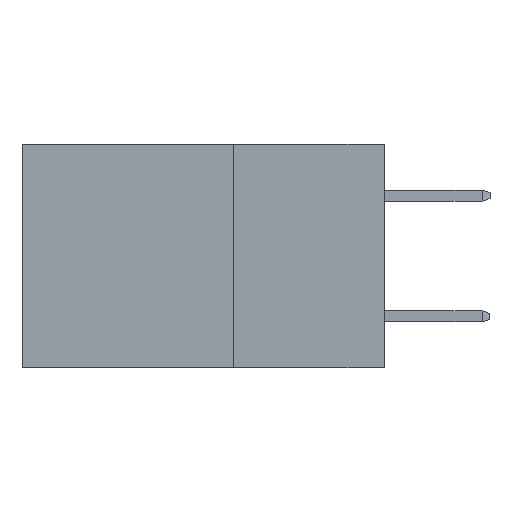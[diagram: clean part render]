
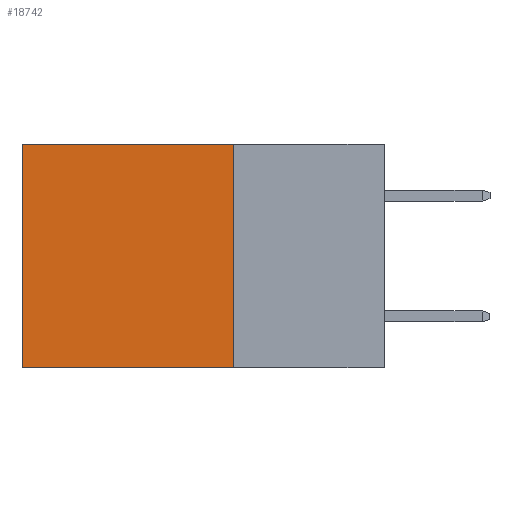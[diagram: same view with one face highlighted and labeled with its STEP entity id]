
A CAD part, left-side view. The second image highlights one B-rep face of the part: STEP entity #18742.
In plain terms, the highlighted planar face has unit normal (-1, 0, 0).
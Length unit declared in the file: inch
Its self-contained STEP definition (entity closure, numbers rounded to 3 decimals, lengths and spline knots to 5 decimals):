
#263 = PLANE ( 'NONE',  #11855 ) ;
#1219 = ORIENTED_EDGE ( 'NONE', *, *, #14883, .T. ) ;
#1270 = EDGE_CURVE ( 'NONE', #6157, #12100, #19484, .T. ) ;
#1410 = DIRECTION ( 'NONE',  ( 0., 1., 0. ) ) ;
#1471 = CARTESIAN_POINT ( 'NONE',  ( 0.298, 0.6, 0. ) ) ;
#1867 = DIRECTION ( 'NONE',  ( 1., 0., 0. ) ) ;
#2210 = VERTEX_POINT ( 'NONE', #16109 ) ;
#2574 = CARTESIAN_POINT ( 'NONE',  ( 0.298, 0.25, -0.37 ) ) ;
#3361 = VECTOR ( 'NONE', #16623, 39.37008 ) ;
#5173 = CARTESIAN_POINT ( 'NONE',  ( 0.298, 0.25, 0. ) ) ;
#6157 = VERTEX_POINT ( 'NONE', #2574 ) ;
#7993 = LINE ( 'NONE', #18135, #11607 ) ;
#8457 = CARTESIAN_POINT ( 'NONE',  ( 0.298, 0.25, -0.37 ) ) ;
#8536 = EDGE_CURVE ( 'NONE', #17518, #2210, #7993, .T. ) ;
#8876 = ORIENTED_EDGE ( 'NONE', *, *, #1270, .F. ) ;
#9138 = VECTOR ( 'NONE', #12306, 39.37008 ) ;
#9176 = CARTESIAN_POINT ( 'NONE',  ( 0.298, 0.25, 0. ) ) ;
#9382 = CARTESIAN_POINT ( 'NONE',  ( 0.298, 0.6, -0.37 ) ) ;
#9492 = CARTESIAN_POINT ( 'NONE',  ( 0.298, 0.25, 0. ) ) ;
#10156 = EDGE_CURVE ( 'NONE', #17518, #6157, #14614, .T. ) ;
#11607 = VECTOR ( 'NONE', #1410, 39.37008 ) ;
#11855 = AXIS2_PLACEMENT_3D ( 'NONE', #9492, #1867, #12614 ) ;
#12100 = VERTEX_POINT ( 'NONE', #9382 ) ;
#12306 = DIRECTION ( 'NONE',  ( 0., 0., -1. ) ) ;
#12614 = DIRECTION ( 'NONE',  ( 0., 0., -1. ) ) ;
#13221 = LINE ( 'NONE', #1471, #9138 ) ;
#14030 = FACE_OUTER_BOUND ( 'NONE', #19691, .T. ) ;
#14614 = LINE ( 'NONE', #9176, #18635 ) ;
#14883 = EDGE_CURVE ( 'NONE', #2210, #12100, #13221, .T. ) ;
#16109 = CARTESIAN_POINT ( 'NONE',  ( 0.298, 0.6, 0. ) ) ;
#16623 = DIRECTION ( 'NONE',  ( 0., 1., 0. ) ) ;
#17033 = ORIENTED_EDGE ( 'NONE', *, *, #10156, .F. ) ;
#17518 = VERTEX_POINT ( 'NONE', #5173 ) ;
#18135 = CARTESIAN_POINT ( 'NONE',  ( 0.298, 0.25, 0. ) ) ;
#18285 = ORIENTED_EDGE ( 'NONE', *, *, #8536, .T. ) ;
#18312 = DIRECTION ( 'NONE',  ( 0., 0., -1. ) ) ;
#18635 = VECTOR ( 'NONE', #18312, 39.37008 ) ;
#18742 = ADVANCED_FACE ( 'NONE', ( #14030 ), #263, .F. ) ;
#19484 = LINE ( 'NONE', #8457, #3361 ) ;
#19691 = EDGE_LOOP ( 'NONE', ( #1219, #8876, #17033, #18285 ) ) ;
